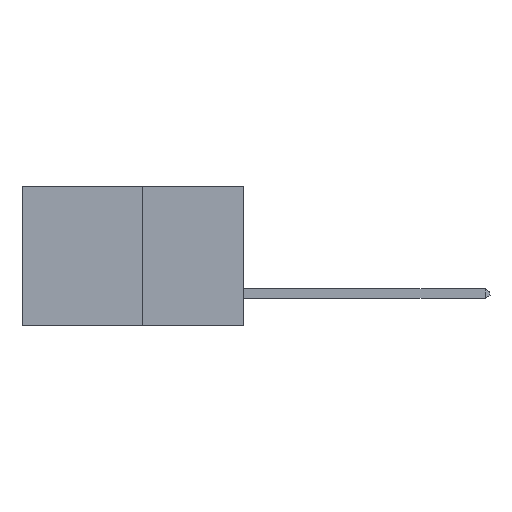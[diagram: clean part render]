
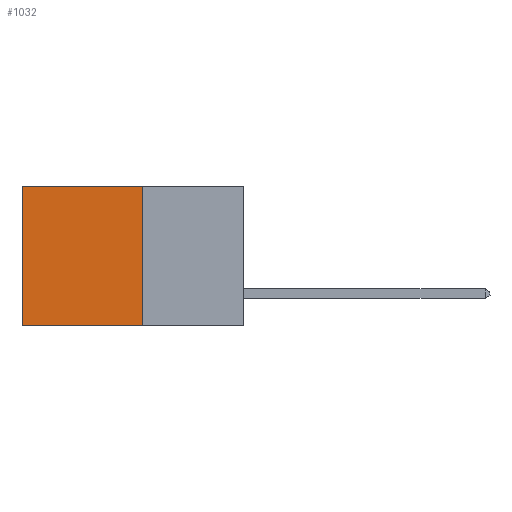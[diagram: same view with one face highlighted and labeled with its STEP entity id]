
A CAD part, left-side view. The second image highlights one B-rep face of the part: STEP entity #1032.
In plain terms, the highlighted planar face has unit normal (-1, 0, 0).
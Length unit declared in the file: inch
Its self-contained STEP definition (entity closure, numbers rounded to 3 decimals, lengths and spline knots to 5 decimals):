
#82 = EDGE_CURVE ( 'NONE', #6585, #6910, #4118, .T. ) ;
#1008 = LINE ( 'NONE', #9286, #3601 ) ;
#1032 = ADVANCED_FACE ( 'NONE', ( #1238 ), #2199, .F. ) ;
#1117 = LINE ( 'NONE', #9069, #1401 ) ;
#1238 = FACE_OUTER_BOUND ( 'NONE', #1418, .T. ) ;
#1309 = VERTEX_POINT ( 'NONE', #9485 ) ;
#1369 = CARTESIAN_POINT ( 'NONE',  ( 0.277, 0.27, 0. ) ) ;
#1401 = VECTOR ( 'NONE', #9053, 39.37008 ) ;
#1418 = EDGE_LOOP ( 'NONE', ( #3761, #3786, #3903, #3970 ) ) ;
#1837 = CARTESIAN_POINT ( 'NONE',  ( 0.277, 0.27, 0. ) ) ;
#2199 = PLANE ( 'NONE',  #5421 ) ;
#2779 = VECTOR ( 'NONE', #5244, 39.37008 ) ;
#3601 = VECTOR ( 'NONE', #9383, 39.37008 ) ;
#3761 = ORIENTED_EDGE ( 'NONE', *, *, #82, .T. ) ;
#3786 = ORIENTED_EDGE ( 'NONE', *, *, #6425, .F. ) ;
#3903 = ORIENTED_EDGE ( 'NONE', *, *, #5334, .F. ) ;
#3916 = VERTEX_POINT ( 'NONE', #1369 ) ;
#3970 = ORIENTED_EDGE ( 'NONE', *, *, #10325, .T. ) ;
#4118 = LINE ( 'NONE', #5210, #4372 ) ;
#4154 = DIRECTION ( 'NONE',  ( 0., 0., -1. ) ) ;
#4281 = DIRECTION ( 'NONE',  ( 1., 0., 0. ) ) ;
#4295 = CARTESIAN_POINT ( 'NONE',  ( 0.277, 0.27, -0.37 ) ) ;
#4372 = VECTOR ( 'NONE', #10754, 39.37008 ) ;
#5094 = CARTESIAN_POINT ( 'NONE',  ( 0.277, 0.59, -0.37 ) ) ;
#5210 = CARTESIAN_POINT ( 'NONE',  ( 0.277, 0.59, -0.37 ) ) ;
#5244 = DIRECTION ( 'NONE',  ( 0., 1., 0. ) ) ;
#5334 = EDGE_CURVE ( 'NONE', #3916, #1309, #1008, .T. ) ;
#5421 = AXIS2_PLACEMENT_3D ( 'NONE', #4295, #4281, #4154 ) ;
#6425 = EDGE_CURVE ( 'NONE', #1309, #6910, #1117, .T. ) ;
#6585 = VERTEX_POINT ( 'NONE', #7636 ) ;
#6910 = VERTEX_POINT ( 'NONE', #5094 ) ;
#7636 = CARTESIAN_POINT ( 'NONE',  ( 0.277, 0.59, 0. ) ) ;
#9053 = DIRECTION ( 'NONE',  ( 0., 1., 0. ) ) ;
#9069 = CARTESIAN_POINT ( 'NONE',  ( 0.277, 0.27, -0.37 ) ) ;
#9286 = CARTESIAN_POINT ( 'NONE',  ( 0.277, 0.27, -0.37 ) ) ;
#9383 = DIRECTION ( 'NONE',  ( 0., 0., -1. ) ) ;
#9485 = CARTESIAN_POINT ( 'NONE',  ( 0.277, 0.27, -0.37 ) ) ;
#9582 = LINE ( 'NONE', #1837, #2779 ) ;
#10325 = EDGE_CURVE ( 'NONE', #3916, #6585, #9582, .T. ) ;
#10754 = DIRECTION ( 'NONE',  ( 0., 0., -1. ) ) ;
